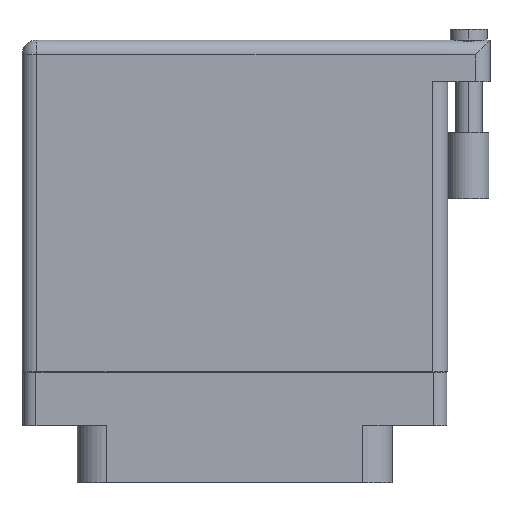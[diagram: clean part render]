
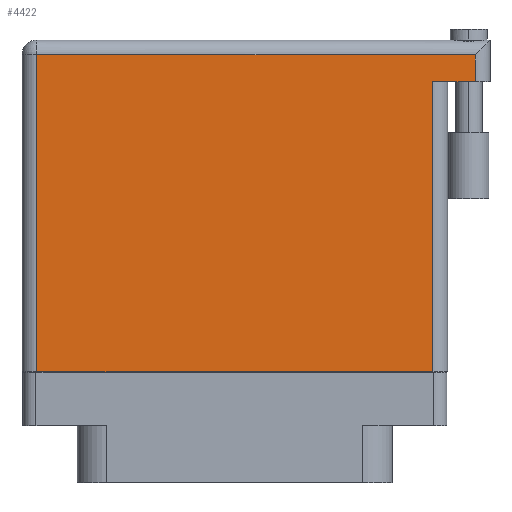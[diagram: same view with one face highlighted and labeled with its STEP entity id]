
A CAD part, front view. The second image highlights one B-rep face of the part: STEP entity #4422.
In plain terms, the highlighted face is planar.
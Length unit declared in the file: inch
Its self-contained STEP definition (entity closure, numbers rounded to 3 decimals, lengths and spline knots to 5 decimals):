
#1087 = DIRECTION ( 'NONE',  ( 0., 0., -1. ) ) ;
#1220 = CARTESIAN_POINT ( 'NONE',  ( -1.004, 1.396, 0.4495 ) ) ;
#1759 = VECTOR ( 'NONE', #26231, 39.37008 ) ;
#1947 = VECTOR ( 'NONE', #21098, 39.37008 ) ;
#2123 = ORIENTED_EDGE ( 'NONE', *, *, #8612, .T. ) ;
#3708 = ORIENTED_EDGE ( 'NONE', *, *, #16638, .F. ) ;
#4422 = ADVANCED_FACE ( 'NONE', ( #32177 ), #20251, .F. ) ;
#4916 = CARTESIAN_POINT ( 'NONE',  ( 1.134, 1.466, 0.4495 ) ) ;
#5761 = LINE ( 'NONE', #28855, #17368 ) ;
#5836 = ORIENTED_EDGE ( 'NONE', *, *, #7563, .T. ) ;
#5927 = CARTESIAN_POINT ( 'NONE',  ( 0.934, 1.269, 0.4495 ) ) ;
#6014 = VECTOR ( 'NONE', #23796, 39.37008 ) ;
#6241 = CARTESIAN_POINT ( 'NONE',  ( -0.934, -0.1, 0.4495 ) ) ;
#6376 = VERTEX_POINT ( 'NONE', #9993 ) ;
#6775 = VERTEX_POINT ( 'NONE', #6241 ) ;
#7563 = EDGE_CURVE ( 'NONE', #21059, #15765, #25202, .T. ) ;
#8159 = LINE ( 'NONE', #34511, #6014 ) ;
#8612 = EDGE_CURVE ( 'NONE', #24771, #11054, #5761, .T. ) ;
#9025 = CARTESIAN_POINT ( 'NONE',  ( 1.134, 1.396, 0.4495 ) ) ;
#9060 = CARTESIAN_POINT ( 'NONE',  ( 0.934, -0.1, 0.4495 ) ) ;
#9993 = CARTESIAN_POINT ( 'NONE',  ( 1.134, 1.269, 0.4495 ) ) ;
#11054 = VERTEX_POINT ( 'NONE', #5927 ) ;
#11705 = EDGE_CURVE ( 'NONE', #6775, #24771, #8159, .T. ) ;
#11722 = DIRECTION ( 'NONE',  ( -1., 0., 0. ) ) ;
#12302 = ORIENTED_EDGE ( 'NONE', *, *, #32780, .T. ) ;
#14369 = LINE ( 'NONE', #4916, #28145 ) ;
#14486 = AXIS2_PLACEMENT_3D ( 'NONE', #33760, #1087, #11722 ) ;
#15463 = VECTOR ( 'NONE', #24646, 39.37008 ) ;
#15765 = VERTEX_POINT ( 'NONE', #24063 ) ;
#16329 = LINE ( 'NONE', #30156, #15463 ) ;
#16638 = EDGE_CURVE ( 'NONE', #6376, #11054, #31491, .T. ) ;
#17368 = VECTOR ( 'NONE', #26452, 39.37008 ) ;
#20251 = PLANE ( 'NONE',  #14486 ) ;
#21059 = VERTEX_POINT ( 'NONE', #9025 ) ;
#21098 = DIRECTION ( 'NONE',  ( -1., 0., 0. ) ) ;
#23796 = DIRECTION ( 'NONE',  ( 1., 0., 0. ) ) ;
#23944 = DIRECTION ( 'NONE',  ( 0., 1., 0. ) ) ;
#24063 = CARTESIAN_POINT ( 'NONE',  ( -0.934, 1.396, 0.4495 ) ) ;
#24646 = DIRECTION ( 'NONE',  ( 0., -1., 0. ) ) ;
#24771 = VERTEX_POINT ( 'NONE', #9060 ) ;
#25202 = LINE ( 'NONE', #1220, #1947 ) ;
#26231 = DIRECTION ( 'NONE',  ( -1., 0., 0. ) ) ;
#26357 = CARTESIAN_POINT ( 'NONE',  ( 1.204, 1.269, 0.4495 ) ) ;
#26452 = DIRECTION ( 'NONE',  ( 0., 1., 0. ) ) ;
#27410 = ORIENTED_EDGE ( 'NONE', *, *, #29699, .T. ) ;
#28145 = VECTOR ( 'NONE', #23944, 39.37008 ) ;
#28567 = ORIENTED_EDGE ( 'NONE', *, *, #11705, .T. ) ;
#28855 = CARTESIAN_POINT ( 'NONE',  ( 0.934, 1.269, 0.4495 ) ) ;
#29699 = EDGE_CURVE ( 'NONE', #15765, #6775, #16329, .T. ) ;
#30156 = CARTESIAN_POINT ( 'NONE',  ( -0.934, -0.1, 0.4495 ) ) ;
#31491 = LINE ( 'NONE', #26357, #1759 ) ;
#32177 = FACE_OUTER_BOUND ( 'NONE', #34366, .T. ) ;
#32780 = EDGE_CURVE ( 'NONE', #6376, #21059, #14369, .T. ) ;
#33760 = CARTESIAN_POINT ( 'NONE',  ( -1.004, 1.466, 0.4495 ) ) ;
#34366 = EDGE_LOOP ( 'NONE', ( #28567, #2123, #3708, #12302, #5836, #27410 ) ) ;
#34511 = CARTESIAN_POINT ( 'NONE',  ( -1.004, -0.1, 0.4495 ) ) ;
